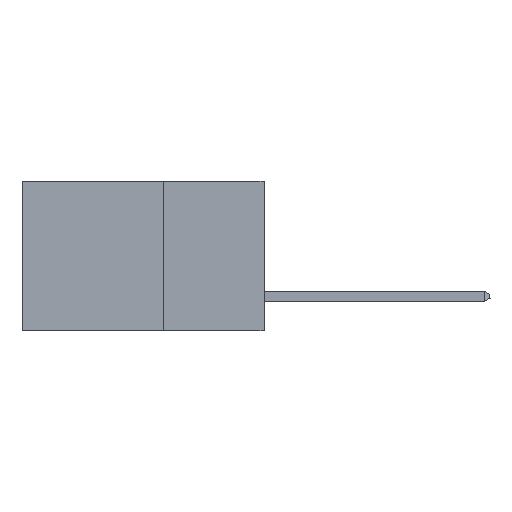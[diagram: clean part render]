
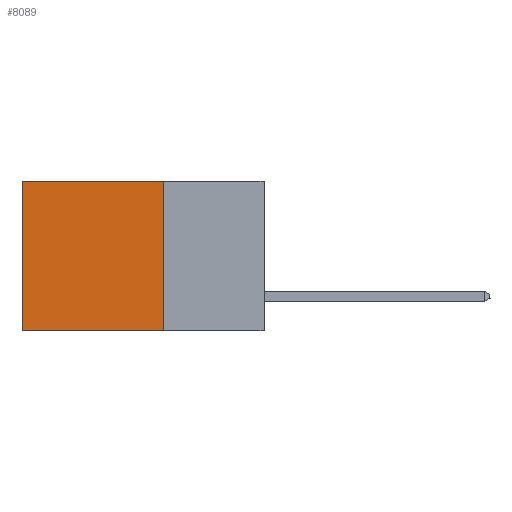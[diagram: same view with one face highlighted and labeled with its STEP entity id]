
A CAD part, left-side view. The second image highlights one B-rep face of the part: STEP entity #8089.
In plain terms, the highlighted planar face has unit normal (-1, 0, 0).
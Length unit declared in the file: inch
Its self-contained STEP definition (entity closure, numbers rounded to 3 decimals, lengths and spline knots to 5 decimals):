
#394 = LINE ( 'NONE', #18977, #20575 ) ;
#960 = FACE_OUTER_BOUND ( 'NONE', #11537, .T. ) ;
#1043 = PLANE ( 'NONE',  #4389 ) ;
#1801 = ORIENTED_EDGE ( 'NONE', *, *, #24383, .F. ) ;
#3054 = CARTESIAN_POINT ( 'NONE',  ( 0.298, 0.6, 0. ) ) ;
#3148 = CARTESIAN_POINT ( 'NONE',  ( 0.298, 0.25, 0. ) ) ;
#3275 = VECTOR ( 'NONE', #23186, 39.37008 ) ;
#4389 = AXIS2_PLACEMENT_3D ( 'NONE', #7252, #9094, #25119 ) ;
#5583 = DIRECTION ( 'NONE',  ( 0., 0., -1. ) ) ;
#6093 = EDGE_CURVE ( 'NONE', #15981, #8349, #14120, .T. ) ;
#7252 = CARTESIAN_POINT ( 'NONE',  ( 0.298, 0.25, 0. ) ) ;
#7592 = VERTEX_POINT ( 'NONE', #13275 ) ;
#8089 = ADVANCED_FACE ( 'NONE', ( #960 ), #1043, .F. ) ;
#8349 = VERTEX_POINT ( 'NONE', #9345 ) ;
#8992 = ORIENTED_EDGE ( 'NONE', *, *, #23751, .T. ) ;
#9094 = DIRECTION ( 'NONE',  ( 1., 0., 0. ) ) ;
#9345 = CARTESIAN_POINT ( 'NONE',  ( 0.298, 0.6, -0.37 ) ) ;
#10408 = ORIENTED_EDGE ( 'NONE', *, *, #6093, .F. ) ;
#11537 = EDGE_LOOP ( 'NONE', ( #17579, #10408, #1801, #8992 ) ) ;
#13275 = CARTESIAN_POINT ( 'NONE',  ( 0.298, 0.25, 0. ) ) ;
#13277 = CARTESIAN_POINT ( 'NONE',  ( 0.298, 0.25, -0.37 ) ) ;
#13356 = DIRECTION ( 'NONE',  ( 0., 0., -1. ) ) ;
#14120 = LINE ( 'NONE', #13277, #3275 ) ;
#14307 = LINE ( 'NONE', #3148, #25153 ) ;
#15499 = VERTEX_POINT ( 'NONE', #3054 ) ;
#15981 = VERTEX_POINT ( 'NONE', #18210 ) ;
#17483 = EDGE_CURVE ( 'NONE', #15499, #8349, #20631, .T. ) ;
#17508 = VECTOR ( 'NONE', #5583, 39.37008 ) ;
#17579 = ORIENTED_EDGE ( 'NONE', *, *, #17483, .T. ) ;
#18210 = CARTESIAN_POINT ( 'NONE',  ( 0.298, 0.25, -0.37 ) ) ;
#18977 = CARTESIAN_POINT ( 'NONE',  ( 0.298, 0.25, 0. ) ) ;
#20575 = VECTOR ( 'NONE', #24737, 39.37008 ) ;
#20631 = LINE ( 'NONE', #21296, #17508 ) ;
#21296 = CARTESIAN_POINT ( 'NONE',  ( 0.298, 0.6, 0. ) ) ;
#23186 = DIRECTION ( 'NONE',  ( 0., 1., 0. ) ) ;
#23751 = EDGE_CURVE ( 'NONE', #7592, #15499, #394, .T. ) ;
#24383 = EDGE_CURVE ( 'NONE', #7592, #15981, #14307, .T. ) ;
#24737 = DIRECTION ( 'NONE',  ( 0., 1., 0. ) ) ;
#25119 = DIRECTION ( 'NONE',  ( 0., 0., -1. ) ) ;
#25153 = VECTOR ( 'NONE', #13356, 39.37008 ) ;
